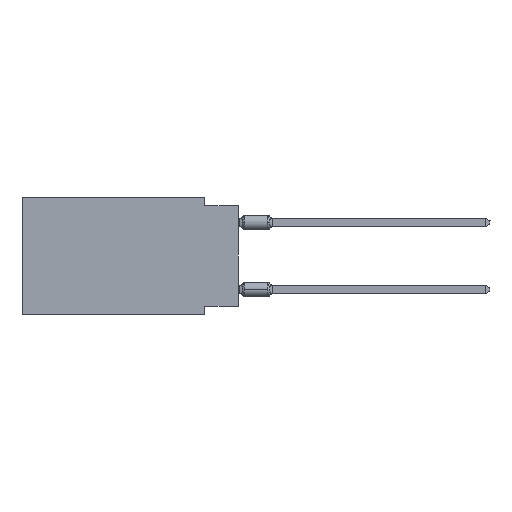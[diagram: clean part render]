
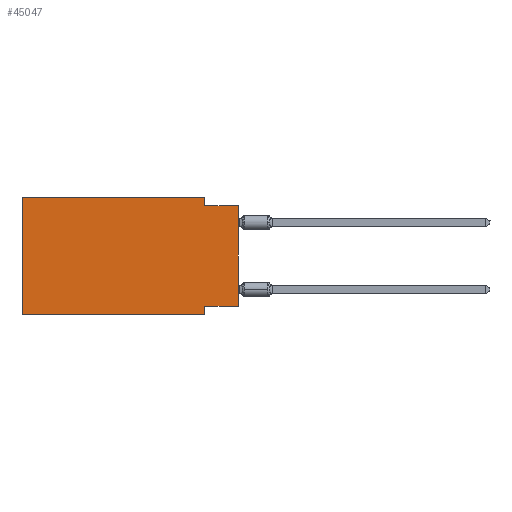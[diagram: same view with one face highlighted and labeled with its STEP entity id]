
A CAD part, left-side view. The second image highlights one B-rep face of the part: STEP entity #45047.
In plain terms, the highlighted planar face has unit normal (-1, 0, 0).
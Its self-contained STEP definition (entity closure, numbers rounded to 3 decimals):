
#656 = LINE ( 'NONE', #40913, #41603 ) ;
#1036 = CARTESIAN_POINT ( 'NONE',  ( 0., 0., 0. ) ) ;
#3819 = CARTESIAN_POINT ( 'NONE',  ( 0., 16.383, -8.89 ) ) ;
#5427 = VERTEX_POINT ( 'NONE', #25939 ) ;
#6264 = DIRECTION ( 'NONE',  ( 0., -1., 0. ) ) ;
#6472 = CARTESIAN_POINT ( 'NONE',  ( 0., 16.383, -8.89 ) ) ;
#6493 = EDGE_CURVE ( 'NONE', #42599, #41048, #65078, .T. ) ;
#7840 = LINE ( 'NONE', #53296, #65195 ) ;
#8104 = DIRECTION ( 'NONE',  ( 0., 1., 0. ) ) ;
#8413 = VERTEX_POINT ( 'NONE', #3819 ) ;
#9000 = VECTOR ( 'NONE', #44047, 1000. ) ;
#12205 = VERTEX_POINT ( 'NONE', #61260 ) ;
#15393 = EDGE_CURVE ( 'NONE', #12205, #42599, #49231, .T. ) ;
#16492 = EDGE_CURVE ( 'NONE', #8413, #48507, #23964, .T. ) ;
#17489 = EDGE_CURVE ( 'NONE', #8413, #18878, #25343, .T. ) ;
#18878 = VERTEX_POINT ( 'NONE', #18953 ) ;
#18953 = CARTESIAN_POINT ( 'NONE',  ( 0., 16.383, 0. ) ) ;
#19234 = EDGE_CURVE ( 'NONE', #5427, #48507, #7840, .T. ) ;
#19636 = CARTESIAN_POINT ( 'NONE',  ( 0., 0., -0.635 ) ) ;
#20397 = CARTESIAN_POINT ( 'NONE',  ( 0., 0., -8.255 ) ) ;
#23782 = DIRECTION ( 'NONE',  ( 0., 0., 1. ) ) ;
#23964 = LINE ( 'NONE', #6472, #25577 ) ;
#24216 = ORIENTED_EDGE ( 'NONE', *, *, #19234, .F. ) ;
#25035 = CARTESIAN_POINT ( 'NONE',  ( 0., 2.54, -8.89 ) ) ;
#25343 = LINE ( 'NONE', #48045, #31662 ) ;
#25577 = VECTOR ( 'NONE', #46679, 1000. ) ;
#25939 = CARTESIAN_POINT ( 'NONE',  ( 0., 2.54, -8.255 ) ) ;
#26738 = VECTOR ( 'NONE', #8104, 1000. ) ;
#27049 = FACE_OUTER_BOUND ( 'NONE', #72055, .T. ) ;
#30469 = VECTOR ( 'NONE', #36786, 1000. ) ;
#30947 = EDGE_CURVE ( 'NONE', #18878, #12205, #656, .T. ) ;
#31222 = LINE ( 'NONE', #20397, #26738 ) ;
#31662 = VECTOR ( 'NONE', #70779, 1000. ) ;
#33383 = DIRECTION ( 'NONE',  ( 1., 0., 0. ) ) ;
#34207 = CARTESIAN_POINT ( 'NONE',  ( 0., 0., -8.255 ) ) ;
#34489 = ORIENTED_EDGE ( 'NONE', *, *, #30947, .F. ) ;
#35672 = CARTESIAN_POINT ( 'NONE',  ( 0., 2.54, -0.635 ) ) ;
#36316 = VECTOR ( 'NONE', #23782, 1000. ) ;
#36786 = DIRECTION ( 'NONE',  ( 0., -1., 0. ) ) ;
#39636 = ORIENTED_EDGE ( 'NONE', *, *, #51556, .T. ) ;
#40242 = AXIS2_PLACEMENT_3D ( 'NONE', #44904, #33383, #49739 ) ;
#40265 = ORIENTED_EDGE ( 'NONE', *, *, #17489, .F. ) ;
#40913 = CARTESIAN_POINT ( 'NONE',  ( 0., 16.383, 0. ) ) ;
#41048 = VERTEX_POINT ( 'NONE', #49950 ) ;
#41603 = VECTOR ( 'NONE', #6264, 1000. ) ;
#42599 = VERTEX_POINT ( 'NONE', #35672 ) ;
#44047 = DIRECTION ( 'NONE',  ( 0., 0., -1. ) ) ;
#44603 = VERTEX_POINT ( 'NONE', #34207 ) ;
#44904 = CARTESIAN_POINT ( 'NONE',  ( 0., 16.383, 0. ) ) ;
#45047 = ADVANCED_FACE ( 'NONE', ( #27049 ), #67602, .F. ) ;
#45873 = DIRECTION ( 'NONE',  ( 0., 0., -1. ) ) ;
#46679 = DIRECTION ( 'NONE',  ( 0., -1., 0. ) ) ;
#48045 = CARTESIAN_POINT ( 'NONE',  ( 0., 16.383, 0. ) ) ;
#48507 = VERTEX_POINT ( 'NONE', #25035 ) ;
#49231 = LINE ( 'NONE', #60784, #9000 ) ;
#49739 = DIRECTION ( 'NONE',  ( 0., 0., -1. ) ) ;
#49950 = CARTESIAN_POINT ( 'NONE',  ( 0., 0., -0.635 ) ) ;
#51556 = EDGE_CURVE ( 'NONE', #44603, #41048, #58765, .T. ) ;
#51669 = ORIENTED_EDGE ( 'NONE', *, *, #6493, .F. ) ;
#53296 = CARTESIAN_POINT ( 'NONE',  ( 0., 2.54, -8.89 ) ) ;
#57039 = ORIENTED_EDGE ( 'NONE', *, *, #16492, .T. ) ;
#57716 = ORIENTED_EDGE ( 'NONE', *, *, #62766, .F. ) ;
#58765 = LINE ( 'NONE', #1036, #36316 ) ;
#60784 = CARTESIAN_POINT ( 'NONE',  ( 0., 2.54, 0. ) ) ;
#61260 = CARTESIAN_POINT ( 'NONE',  ( 0., 2.54, 0. ) ) ;
#62766 = EDGE_CURVE ( 'NONE', #44603, #5427, #31222, .T. ) ;
#63329 = ORIENTED_EDGE ( 'NONE', *, *, #15393, .F. ) ;
#65078 = LINE ( 'NONE', #19636, #30469 ) ;
#65195 = VECTOR ( 'NONE', #45873, 1000. ) ;
#67602 = PLANE ( 'NONE',  #40242 ) ;
#70779 = DIRECTION ( 'NONE',  ( 0., 0., 1. ) ) ;
#72055 = EDGE_LOOP ( 'NONE', ( #39636, #51669, #63329, #34489, #40265, #57039, #24216, #57716 ) ) ;
